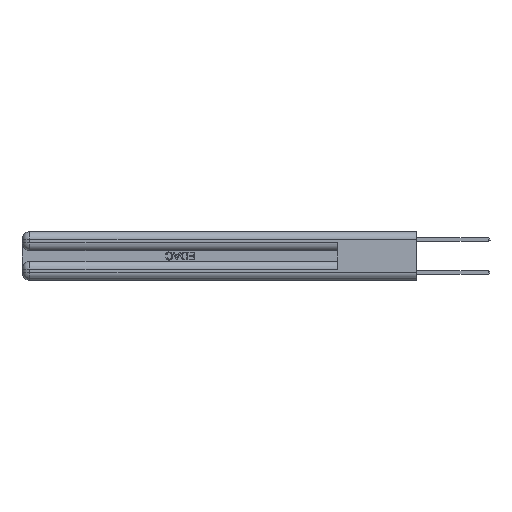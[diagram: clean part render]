
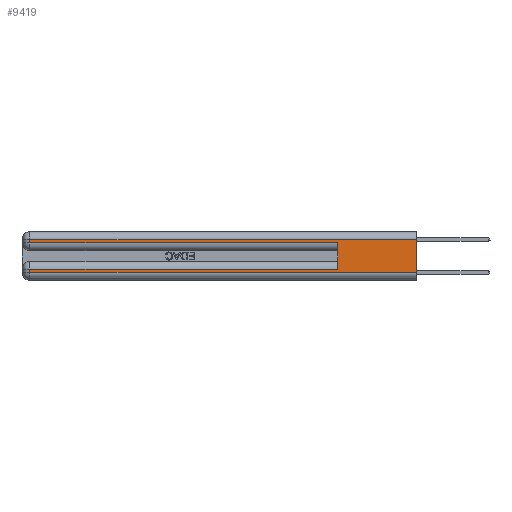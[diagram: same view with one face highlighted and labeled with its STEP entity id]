
A CAD part, left-side view. The second image highlights one B-rep face of the part: STEP entity #9419.
In plain terms, the highlighted planar face has unit normal (-1, 0, 0).
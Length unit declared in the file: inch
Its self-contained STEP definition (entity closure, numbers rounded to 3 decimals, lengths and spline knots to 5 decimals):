
#310 = VERTEX_POINT ( 'NONE', #22648 ) ;
#740 = ORIENTED_EDGE ( 'NONE', *, *, #16200, .F. ) ;
#898 = AXIS2_PLACEMENT_3D ( 'NONE', #23949, #19195, #24146 ) ;
#1208 = VERTEX_POINT ( 'NONE', #21388 ) ;
#1959 = VERTEX_POINT ( 'NONE', #4307 ) ;
#2020 = ORIENTED_EDGE ( 'NONE', *, *, #32778, .T. ) ;
#2505 = LINE ( 'NONE', #6339, #30117 ) ;
#2993 = DIRECTION ( 'NONE',  ( 0., 0., 1. ) ) ;
#3276 = EDGE_CURVE ( 'NONE', #22812, #11283, #14194, .T. ) ;
#3416 = EDGE_CURVE ( 'NONE', #1959, #10743, #10901, .T. ) ;
#4048 = VECTOR ( 'NONE', #33439, 39.37008 ) ;
#4307 = CARTESIAN_POINT ( 'NONE',  ( 0., 2.94, 0.31 ) ) ;
#5120 = DIRECTION ( 'NONE',  ( 0., -1., 0. ) ) ;
#5539 = DIRECTION ( 'NONE',  ( 0., 0., -1. ) ) ;
#5793 = PLANE ( 'NONE',  #898 ) ;
#6339 = CARTESIAN_POINT ( 'NONE',  ( 0., 0., 0.085 ) ) ;
#7191 = LINE ( 'NONE', #20288, #27088 ) ;
#7664 = VERTEX_POINT ( 'NONE', #23780 ) ;
#8311 = CARTESIAN_POINT ( 'NONE',  ( 0., 2.94, 0.085 ) ) ;
#8629 = CARTESIAN_POINT ( 'NONE',  ( 0., 2.94, 0.285 ) ) ;
#8903 = ORIENTED_EDGE ( 'NONE', *, *, #20211, .F. ) ;
#9419 = ADVANCED_FACE ( 'NONE', ( #23142 ), #5793, .F. ) ;
#9685 = DIRECTION ( 'NONE',  ( 0., 1., 0. ) ) ;
#10072 = ORIENTED_EDGE ( 'NONE', *, *, #3276, .T. ) ;
#10432 = CARTESIAN_POINT ( 'NONE',  ( 0., 0., 0.285 ) ) ;
#10743 = VERTEX_POINT ( 'NONE', #8629 ) ;
#10901 = LINE ( 'NONE', #15168, #4048 ) ;
#10966 = CARTESIAN_POINT ( 'NONE',  ( 0., 0., 0.37 ) ) ;
#11283 = VERTEX_POINT ( 'NONE', #21485 ) ;
#11713 = ORIENTED_EDGE ( 'NONE', *, *, #25861, .T. ) ;
#12343 = LINE ( 'NONE', #33125, #15576 ) ;
#13733 = EDGE_LOOP ( 'NONE', ( #8903, #11713, #29936, #30754, #740, #14539, #10072, #2020 ) ) ;
#14194 = LINE ( 'NONE', #29841, #15802 ) ;
#14539 = ORIENTED_EDGE ( 'NONE', *, *, #29303, .T. ) ;
#15100 = DIRECTION ( 'NONE',  ( 0., -1., 0. ) ) ;
#15168 = CARTESIAN_POINT ( 'NONE',  ( 0., 2.94, 0.37 ) ) ;
#15576 = VECTOR ( 'NONE', #15100, 39.37008 ) ;
#15620 = CARTESIAN_POINT ( 'NONE',  ( 0., 0.6, 0.145 ) ) ;
#15802 = VECTOR ( 'NONE', #21777, 39.37008 ) ;
#16200 = EDGE_CURVE ( 'NONE', #21856, #1208, #28688, .T. ) ;
#18126 = VECTOR ( 'NONE', #5539, 39.37008 ) ;
#19195 = DIRECTION ( 'NONE',  ( 1., 0., 0. ) ) ;
#20211 = EDGE_CURVE ( 'NONE', #310, #7664, #24227, .T. ) ;
#20288 = CARTESIAN_POINT ( 'NONE',  ( 0., 0., 0.31 ) ) ;
#21388 = CARTESIAN_POINT ( 'NONE',  ( 0., 0.6, 0.285 ) ) ;
#21485 = CARTESIAN_POINT ( 'NONE',  ( 0., 2.94, 0.06 ) ) ;
#21777 = DIRECTION ( 'NONE',  ( 0., 0., -1. ) ) ;
#21856 = VERTEX_POINT ( 'NONE', #25181 ) ;
#22225 = DIRECTION ( 'NONE',  ( 0., 1., 0. ) ) ;
#22648 = CARTESIAN_POINT ( 'NONE',  ( 0., 0., 0.31 ) ) ;
#22812 = VERTEX_POINT ( 'NONE', #8311 ) ;
#23142 = FACE_OUTER_BOUND ( 'NONE', #13733, .T. ) ;
#23739 = LINE ( 'NONE', #10432, #24959 ) ;
#23780 = CARTESIAN_POINT ( 'NONE',  ( 0., 0., 0.06 ) ) ;
#23949 = CARTESIAN_POINT ( 'NONE',  ( 0., 0., 0.37 ) ) ;
#24146 = DIRECTION ( 'NONE',  ( 0., 0., -1. ) ) ;
#24227 = LINE ( 'NONE', #10966, #18126 ) ;
#24959 = VECTOR ( 'NONE', #5120, 39.37008 ) ;
#25181 = CARTESIAN_POINT ( 'NONE',  ( 0., 0.6, 0.085 ) ) ;
#25861 = EDGE_CURVE ( 'NONE', #310, #1959, #7191, .T. ) ;
#27088 = VECTOR ( 'NONE', #9685, 39.37008 ) ;
#28688 = LINE ( 'NONE', #15620, #30345 ) ;
#29303 = EDGE_CURVE ( 'NONE', #21856, #22812, #2505, .T. ) ;
#29841 = CARTESIAN_POINT ( 'NONE',  ( 0., 2.94, 0.37 ) ) ;
#29936 = ORIENTED_EDGE ( 'NONE', *, *, #3416, .T. ) ;
#30117 = VECTOR ( 'NONE', #22225, 39.37008 ) ;
#30345 = VECTOR ( 'NONE', #2993, 39.37008 ) ;
#30754 = ORIENTED_EDGE ( 'NONE', *, *, #32868, .T. ) ;
#32778 = EDGE_CURVE ( 'NONE', #11283, #7664, #12343, .T. ) ;
#32868 = EDGE_CURVE ( 'NONE', #10743, #1208, #23739, .T. ) ;
#33125 = CARTESIAN_POINT ( 'NONE',  ( 0., 0., 0.06 ) ) ;
#33439 = DIRECTION ( 'NONE',  ( 0., 0., -1. ) ) ;
